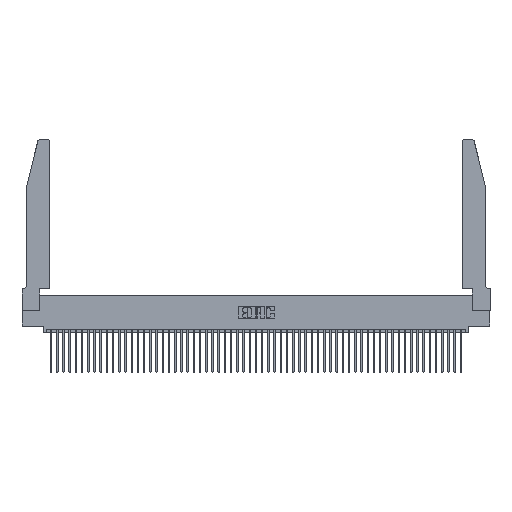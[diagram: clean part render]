
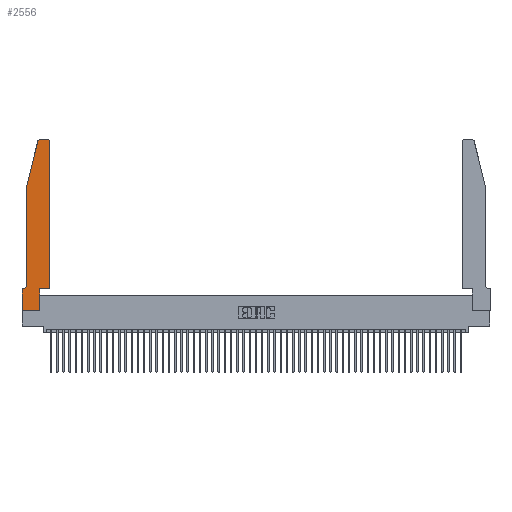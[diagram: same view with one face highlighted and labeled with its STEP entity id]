
A CAD part, top view. The second image highlights one B-rep face of the part: STEP entity #2556.
In plain terms, the highlighted planar face has unit normal (0, 0, 1).
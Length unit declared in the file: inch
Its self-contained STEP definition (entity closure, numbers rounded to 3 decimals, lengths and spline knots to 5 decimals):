
#14 = CARTESIAN_POINT ( 'NONE',  ( 0.0055, 0.42, 0.37 ) ) ;
#1866 = VERTEX_POINT ( 'NONE', #8532 ) ;
#2038 = CARTESIAN_POINT ( 'NONE',  ( 0.0755, 2., 0.37 ) ) ;
#2556 = ADVANCED_FACE ( 'NONE', ( #18828 ), #44969, .T. ) ;
#2733 = VERTEX_POINT ( 'NONE', #16387 ) ;
#3147 = CARTESIAN_POINT ( 'NONE',  ( 0.0055, 0.35, 0.37 ) ) ;
#5447 = DIRECTION ( 'NONE',  ( 1., 0., 0. ) ) ;
#6928 = ORIENTED_EDGE ( 'NONE', *, *, #8226, .T. ) ;
#7066 = CARTESIAN_POINT ( 'NONE',  ( 0.4505, 0.35, 0.37 ) ) ;
#7838 = DIRECTION ( 'NONE',  ( -1., 0., 0. ) ) ;
#8226 = EDGE_CURVE ( 'NONE', #22635, #12171, #52504, .T. ) ;
#8532 = CARTESIAN_POINT ( 'NONE',  ( 0.4505, 2.72, 0.37 ) ) ;
#9715 = AXIS2_PLACEMENT_3D ( 'NONE', #13213, #42450, #13041 ) ;
#9733 = LINE ( 'NONE', #33965, #45718 ) ;
#10402 = CARTESIAN_POINT ( 'NONE',  ( 0.2865, 0., 0.37 ) ) ;
#10877 = CARTESIAN_POINT ( 'NONE',  ( 0., 0., 0.37 ) ) ;
#10901 = AXIS2_PLACEMENT_3D ( 'NONE', #53733, #32528, #15903 ) ;
#10953 = DIRECTION ( 'NONE',  ( 0., -1., 0. ) ) ;
#12171 = VERTEX_POINT ( 'NONE', #32857 ) ;
#12306 = ORIENTED_EDGE ( 'NONE', *, *, #52550, .T. ) ;
#13041 = DIRECTION ( 'NONE',  ( 1., 0., 0. ) ) ;
#13213 = CARTESIAN_POINT ( 'NONE',  ( 0.4205, 2.72, 0.37 ) ) ;
#13847 = EDGE_CURVE ( 'NONE', #31136, #1866, #33654, .T. ) ;
#14923 = DIRECTION ( 'NONE',  ( 0., 0., 1. ) ) ;
#15347 = CARTESIAN_POINT ( 'NONE',  ( 0.0755, 2., 0.37 ) ) ;
#15445 = DIRECTION ( 'NONE',  ( 1., 0., 0. ) ) ;
#15903 = DIRECTION ( 'NONE',  ( 1., 0., 0. ) ) ;
#16387 = CARTESIAN_POINT ( 'NONE',  ( 0.4205, 2.75, 0.37 ) ) ;
#16701 = CIRCLE ( 'NONE', #9715, 0.03 ) ;
#17752 = EDGE_CURVE ( 'NONE', #51854, #47599, #18194, .T. ) ;
#17764 = VECTOR ( 'NONE', #5447, 39.37008 ) ;
#18194 = CIRCLE ( 'NONE', #18531, 0.07 ) ;
#18531 = AXIS2_PLACEMENT_3D ( 'NONE', #14, #20314, #7838 ) ;
#18664 = EDGE_CURVE ( 'NONE', #52498, #51854, #29178, .T. ) ;
#18753 = ORIENTED_EDGE ( 'NONE', *, *, #35238, .T. ) ;
#18828 = FACE_OUTER_BOUND ( 'NONE', #38489, .T. ) ;
#20314 = DIRECTION ( 'NONE',  ( 0., 0., -1. ) ) ;
#20389 = AXIS2_PLACEMENT_3D ( 'NONE', #23317, #14923, #35578 ) ;
#22538 = ORIENTED_EDGE ( 'NONE', *, *, #22919, .T. ) ;
#22635 = VERTEX_POINT ( 'NONE', #25866 ) ;
#22765 = ORIENTED_EDGE ( 'NONE', *, *, #39646, .T. ) ;
#22919 = EDGE_CURVE ( 'NONE', #32619, #42186, #53564, .T. ) ;
#23317 = CARTESIAN_POINT ( 'NONE',  ( 0.284, 2.72, 0.37 ) ) ;
#23740 = ORIENTED_EDGE ( 'NONE', *, *, #13847, .T. ) ;
#24829 = CARTESIAN_POINT ( 'NONE',  ( 0., 0.35, 0.37 ) ) ;
#25866 = CARTESIAN_POINT ( 'NONE',  ( 0.284, 2.75, 0.37 ) ) ;
#27205 = EDGE_CURVE ( 'NONE', #47599, #32619, #44668, .T. ) ;
#28100 = VERTEX_POINT ( 'NONE', #43612 ) ;
#28252 = DIRECTION ( 'NONE',  ( 0., -1., 0. ) ) ;
#28962 = VECTOR ( 'NONE', #40784, 39.37008 ) ;
#29178 = LINE ( 'NONE', #15347, #29802 ) ;
#29552 = VERTEX_POINT ( 'NONE', #10402 ) ;
#29751 = EDGE_CURVE ( 'NONE', #12171, #52498, #9733, .T. ) ;
#29802 = VECTOR ( 'NONE', #10953, 39.37008 ) ;
#29980 = VECTOR ( 'NONE', #28252, 39.37008 ) ;
#30078 = ORIENTED_EDGE ( 'NONE', *, *, #27205, .T. ) ;
#30087 = EDGE_CURVE ( 'NONE', #2733, #22635, #43798, .T. ) ;
#31136 = VERTEX_POINT ( 'NONE', #7066 ) ;
#31304 = VECTOR ( 'NONE', #40503, 39.37008 ) ;
#31599 = CARTESIAN_POINT ( 'NONE',  ( 0.2865, 0.35, 0.37 ) ) ;
#32528 = DIRECTION ( 'NONE',  ( 0., 0., 1. ) ) ;
#32619 = VERTEX_POINT ( 'NONE', #24829 ) ;
#32857 = CARTESIAN_POINT ( 'NONE',  ( 0.25487, 2.72718, 0.37 ) ) ;
#33025 = DIRECTION ( 'NONE',  ( -0.239, -0.971, 0. ) ) ;
#33654 = LINE ( 'NONE', #40207, #51342 ) ;
#33965 = CARTESIAN_POINT ( 'NONE',  ( 0.0755, 2., 0.37 ) ) ;
#34025 = CARTESIAN_POINT ( 'NONE',  ( 0.0755, 0.42, 0.37 ) ) ;
#35238 = EDGE_CURVE ( 'NONE', #42186, #29552, #53671, .T. ) ;
#35363 = VECTOR ( 'NONE', #15445, 39.37008 ) ;
#35578 = DIRECTION ( 'NONE',  ( 1., 0., 0. ) ) ;
#37800 = CARTESIAN_POINT ( 'NONE',  ( 0., 0., 0.37 ) ) ;
#38016 = LINE ( 'NONE', #47473, #17764 ) ;
#38489 = EDGE_LOOP ( 'NONE', ( #46700, #6928, #45872, #46252, #45183, #30078, #22538, #18753, #12306, #22765, #23740, #45092 ) ) ;
#39646 = EDGE_CURVE ( 'NONE', #28100, #31136, #38016, .T. ) ;
#40207 = CARTESIAN_POINT ( 'NONE',  ( 0.4505, 0.35, 0.37 ) ) ;
#40503 = DIRECTION ( 'NONE',  ( -1., 0., 0. ) ) ;
#40784 = DIRECTION ( 'NONE',  ( -1., 0., 0. ) ) ;
#42186 = VERTEX_POINT ( 'NONE', #37800 ) ;
#42450 = DIRECTION ( 'NONE',  ( 0., 0., 1. ) ) ;
#43612 = CARTESIAN_POINT ( 'NONE',  ( 0.2865, 0.35, 0.37 ) ) ;
#43798 = LINE ( 'NONE', #44167, #31304 ) ;
#44167 = CARTESIAN_POINT ( 'NONE',  ( 0.2605, 2.75, 0.37 ) ) ;
#44668 = LINE ( 'NONE', #53749, #28962 ) ;
#44969 = PLANE ( 'NONE',  #10901 ) ;
#45063 = VECTOR ( 'NONE', #48226, 39.37008 ) ;
#45092 = ORIENTED_EDGE ( 'NONE', *, *, #47381, .T. ) ;
#45183 = ORIENTED_EDGE ( 'NONE', *, *, #17752, .T. ) ;
#45718 = VECTOR ( 'NONE', #33025, 39.37008 ) ;
#45872 = ORIENTED_EDGE ( 'NONE', *, *, #29751, .T. ) ;
#46252 = ORIENTED_EDGE ( 'NONE', *, *, #18664, .T. ) ;
#46345 = LINE ( 'NONE', #31599, #45063 ) ;
#46700 = ORIENTED_EDGE ( 'NONE', *, *, #30087, .T. ) ;
#47381 = EDGE_CURVE ( 'NONE', #1866, #2733, #16701, .T. ) ;
#47473 = CARTESIAN_POINT ( 'NONE',  ( 0.4505, 0.35, 0.37 ) ) ;
#47599 = VERTEX_POINT ( 'NONE', #3147 ) ;
#48226 = DIRECTION ( 'NONE',  ( 0., 1., 0. ) ) ;
#48745 = CARTESIAN_POINT ( 'NONE',  ( 0., 0., 0.37 ) ) ;
#48784 = DIRECTION ( 'NONE',  ( 0., 1., 0. ) ) ;
#51342 = VECTOR ( 'NONE', #48784, 39.37008 ) ;
#51854 = VERTEX_POINT ( 'NONE', #34025 ) ;
#52498 = VERTEX_POINT ( 'NONE', #2038 ) ;
#52504 = CIRCLE ( 'NONE', #20389, 0.03 ) ;
#52550 = EDGE_CURVE ( 'NONE', #29552, #28100, #46345, .T. ) ;
#53564 = LINE ( 'NONE', #48745, #29980 ) ;
#53671 = LINE ( 'NONE', #10877, #35363 ) ;
#53733 = CARTESIAN_POINT ( 'NONE',  ( 0., 0.35, 0.37 ) ) ;
#53749 = CARTESIAN_POINT ( 'NONE',  ( 0.0755, 0.35, 0.37 ) ) ;
